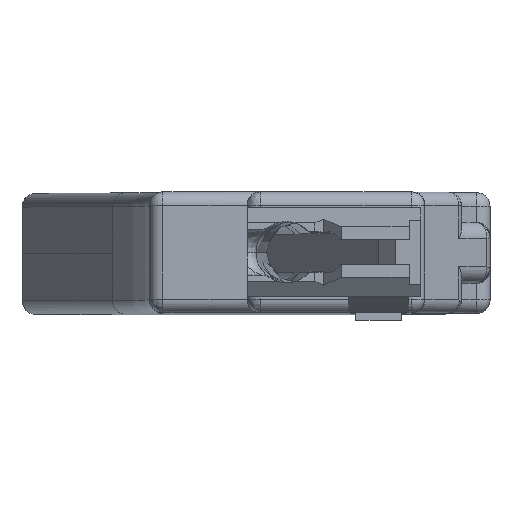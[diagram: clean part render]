
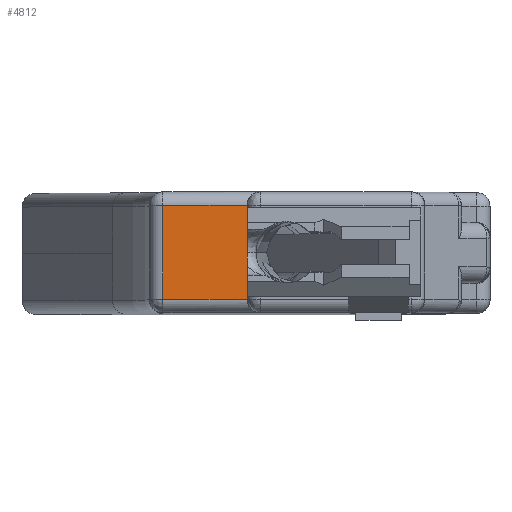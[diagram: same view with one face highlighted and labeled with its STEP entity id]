
A CAD part, top view. The second image highlights one B-rep face of the part: STEP entity #4812.
In plain terms, the highlighted planar face has unit normal (0, 0, 1).
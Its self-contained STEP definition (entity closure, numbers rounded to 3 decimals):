
#747=FACE_OUTER_BOUND('',#1039,.T.);
#1039=EDGE_LOOP('',(#4302,#4303,#4304,#4305));
#1206=LINE('',#9079,#1500);
#1319=LINE('',#11572,#1613);
#1351=LINE('',#11695,#1645);
#1352=LINE('',#11697,#1646);
#1500=VECTOR('',#5744,10.);
#1613=VECTOR('',#6195,10.);
#1645=VECTOR('',#6295,10.);
#1646=VECTOR('',#6298,10.);
#2012=VERTEX_POINT('',#8879);
#2039=VERTEX_POINT('',#9075);
#2218=VERTEX_POINT('',#11571);
#2241=VERTEX_POINT('',#11693);
#2593=EDGE_CURVE('',#2012,#2039,#1206,.T.);
#2898=EDGE_CURVE('',#2039,#2218,#1319,.T.);
#2946=EDGE_CURVE('',#2012,#2241,#1351,.T.);
#2947=EDGE_CURVE('',#2218,#2241,#1352,.T.);
#4302=ORIENTED_EDGE('',*,*,#2898,.F.);
#4303=ORIENTED_EDGE('',*,*,#2593,.F.);
#4304=ORIENTED_EDGE('',*,*,#2946,.T.);
#4305=ORIENTED_EDGE('',*,*,#2947,.F.);
#4543=PLANE('',#5225);
#4812=ADVANCED_FACE('',(#747),#4543,.F.);
#5225=AXIS2_PLACEMENT_3D('',#11696,#6296,#6297);
#5744=DIRECTION('',(-1.,0.,0.));
#6195=DIRECTION('',(0.,1.,0.));
#6295=DIRECTION('',(0.,1.,0.));
#6296=DIRECTION('center_axis',(0.,0.,
-1.));
#6297=DIRECTION('ref_axis',(-1.,0.,0.));
#6298=DIRECTION('',(1.,0.,0.));
#8879=CARTESIAN_POINT('',(864.104,14.622,210.987));
#9075=CARTESIAN_POINT('',(848.604,14.622,210.987));
#9079=CARTESIAN_POINT('',(862.777,14.622,210.987));
#11571=CARTESIAN_POINT('',(848.604,31.923,210.987));
#11572=CARTESIAN_POINT('',(848.604,19.168,210.987));
#11693=CARTESIAN_POINT('',(864.104,31.923,210.987));
#11695=CARTESIAN_POINT('',(864.104,15.063,210.987));
#11696=CARTESIAN_POINT('Origin',(864.104,15.063,210.987));
#11697=CARTESIAN_POINT('',(883.864,31.923,210.987));
